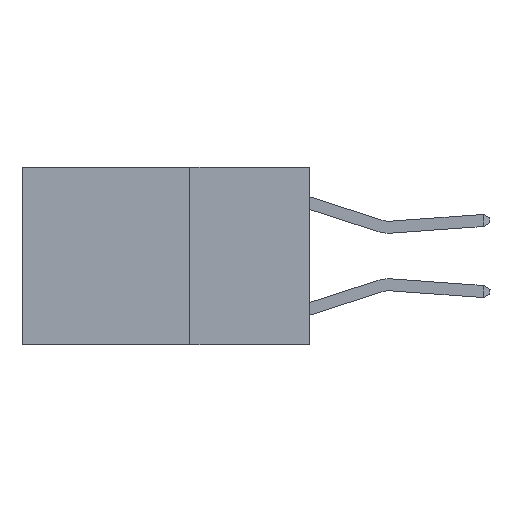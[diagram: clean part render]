
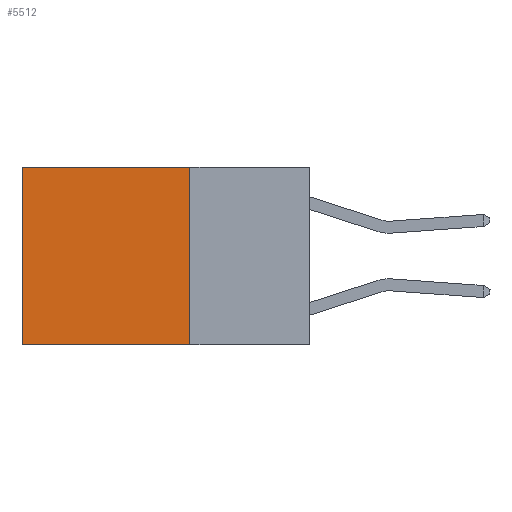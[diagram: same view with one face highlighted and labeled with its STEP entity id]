
A CAD part, left-side view. The second image highlights one B-rep face of the part: STEP entity #5512.
In plain terms, the highlighted planar face has unit normal (-1, 0, 0).
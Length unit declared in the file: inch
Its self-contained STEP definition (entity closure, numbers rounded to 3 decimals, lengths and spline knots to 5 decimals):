
#658 = CARTESIAN_POINT ( 'NONE',  ( 0.2625, 0.25, 0. ) ) ;
#2707 = PLANE ( 'NONE',  #15263 ) ;
#3376 = ORIENTED_EDGE ( 'NONE', *, *, #18443, .T. ) ;
#3637 = ORIENTED_EDGE ( 'NONE', *, *, #13388, .F. ) ;
#3797 = VECTOR ( 'NONE', #11970, 39.37008 ) ;
#5512 = ADVANCED_FACE ( 'NONE', ( #6797 ), #2707, .F. ) ;
#6797 = FACE_OUTER_BOUND ( 'NONE', #14827, .T. ) ;
#8211 = DIRECTION ( 'NONE',  ( 0., 1., 0. ) ) ;
#8978 = DIRECTION ( 'NONE',  ( 1., 0., 0. ) ) ;
#9058 = DIRECTION ( 'NONE',  ( 0., 0., -1. ) ) ;
#9711 = CARTESIAN_POINT ( 'NONE',  ( 0.2625, 0.25, -0.37 ) ) ;
#10127 = LINE ( 'NONE', #22805, #16845 ) ;
#10429 = VERTEX_POINT ( 'NONE', #16079 ) ;
#11093 = CARTESIAN_POINT ( 'NONE',  ( 0.2625, 0.25, 0. ) ) ;
#11970 = DIRECTION ( 'NONE',  ( 0., 1., 0. ) ) ;
#12229 = LINE ( 'NONE', #26530, #3797 ) ;
#13388 = EDGE_CURVE ( 'NONE', #10429, #18894, #14223, .T. ) ;
#13778 = ORIENTED_EDGE ( 'NONE', *, *, #26491, .F. ) ;
#14223 = LINE ( 'NONE', #9711, #19799 ) ;
#14827 = EDGE_LOOP ( 'NONE', ( #24607, #3637, #13778, #3376 ) ) ;
#15263 = AXIS2_PLACEMENT_3D ( 'NONE', #658, #8978, #17318 ) ;
#16025 = DIRECTION ( 'NONE',  ( 0., 0., -1. ) ) ;
#16079 = CARTESIAN_POINT ( 'NONE',  ( 0.2625, 0.25, -0.37 ) ) ;
#16845 = VECTOR ( 'NONE', #16025, 39.37008 ) ;
#17219 = VERTEX_POINT ( 'NONE', #25254 ) ;
#17318 = DIRECTION ( 'NONE',  ( 0., 0., -1. ) ) ;
#17791 = LINE ( 'NONE', #11093, #21006 ) ;
#18443 = EDGE_CURVE ( 'NONE', #17219, #23386, #12229, .T. ) ;
#18894 = VERTEX_POINT ( 'NONE', #21890 ) ;
#19799 = VECTOR ( 'NONE', #8211, 39.37008 ) ;
#21006 = VECTOR ( 'NONE', #9058, 39.37008 ) ;
#21890 = CARTESIAN_POINT ( 'NONE',  ( 0.2625, 0.6, -0.37 ) ) ;
#22287 = EDGE_CURVE ( 'NONE', #23386, #18894, #10127, .T. ) ;
#22805 = CARTESIAN_POINT ( 'NONE',  ( 0.2625, 0.6, 0. ) ) ;
#23386 = VERTEX_POINT ( 'NONE', #23795 ) ;
#23795 = CARTESIAN_POINT ( 'NONE',  ( 0.2625, 0.6, 0. ) ) ;
#24607 = ORIENTED_EDGE ( 'NONE', *, *, #22287, .T. ) ;
#25254 = CARTESIAN_POINT ( 'NONE',  ( 0.2625, 0.25, 0. ) ) ;
#26491 = EDGE_CURVE ( 'NONE', #17219, #10429, #17791, .T. ) ;
#26530 = CARTESIAN_POINT ( 'NONE',  ( 0.2625, 0.25, 0. ) ) ;
